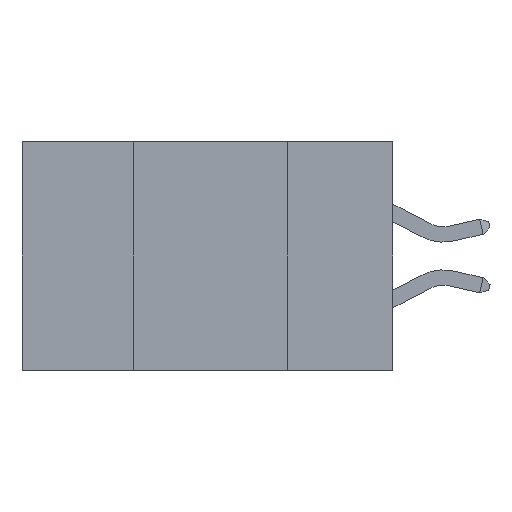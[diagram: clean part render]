
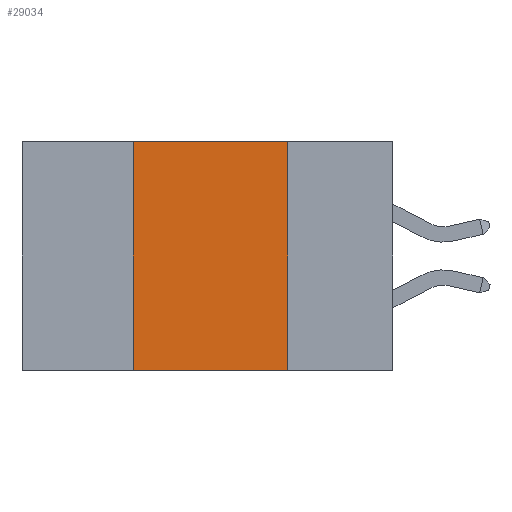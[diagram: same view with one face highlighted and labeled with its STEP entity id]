
A CAD part, left-side view. The second image highlights one B-rep face of the part: STEP entity #29034.
In plain terms, the highlighted planar face has unit normal (-1, 0, 0).
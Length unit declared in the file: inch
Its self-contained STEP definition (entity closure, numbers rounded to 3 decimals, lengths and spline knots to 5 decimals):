
#179 = CARTESIAN_POINT ( 'NONE',  ( 0., 0.17, 0. ) ) ;
#1190 = ORIENTED_EDGE ( 'NONE', *, *, #21436, .F. ) ;
#2855 = CARTESIAN_POINT ( 'NONE',  ( 0., 0.42, -0.37 ) ) ;
#4758 = CARTESIAN_POINT ( 'NONE',  ( 0., 0.6, 0. ) ) ;
#5437 = DIRECTION ( 'NONE',  ( 0., 0., -1. ) ) ;
#5873 = DIRECTION ( 'NONE',  ( 0., -1., 0. ) ) ;
#6103 = CARTESIAN_POINT ( 'NONE',  ( 0., 0.17, 0. ) ) ;
#6507 = VECTOR ( 'NONE', #5437, 39.37008 ) ;
#7411 = LINE ( 'NONE', #17559, #20046 ) ;
#9074 = ORIENTED_EDGE ( 'NONE', *, *, #22148, .F. ) ;
#9083 = ORIENTED_EDGE ( 'NONE', *, *, #24152, .F. ) ;
#9191 = AXIS2_PLACEMENT_3D ( 'NONE', #4758, #12447, #14765 ) ;
#10175 = LINE ( 'NONE', #15884, #22792 ) ;
#12447 = DIRECTION ( 'NONE',  ( 1., 0., 0. ) ) ;
#12981 = CARTESIAN_POINT ( 'NONE',  ( 0., 0.6, -0.37 ) ) ;
#13881 = VERTEX_POINT ( 'NONE', #2855 ) ;
#14174 = CARTESIAN_POINT ( 'NONE',  ( 0., 0.42, 0. ) ) ;
#14760 = LINE ( 'NONE', #179, #6507 ) ;
#14765 = DIRECTION ( 'NONE',  ( 0., 0., -1. ) ) ;
#14948 = EDGE_LOOP ( 'NONE', ( #9083, #9074, #1190, #19079 ) ) ;
#15280 = EDGE_CURVE ( 'NONE', #13881, #19726, #16064, .T. ) ;
#15884 = CARTESIAN_POINT ( 'NONE',  ( 0., 0.42, 0. ) ) ;
#16064 = LINE ( 'NONE', #12981, #19278 ) ;
#17559 = CARTESIAN_POINT ( 'NONE',  ( 0., 0.6, 0. ) ) ;
#19079 = ORIENTED_EDGE ( 'NONE', *, *, #15280, .T. ) ;
#19278 = VECTOR ( 'NONE', #25984, 39.37008 ) ;
#19669 = CARTESIAN_POINT ( 'NONE',  ( 0., 0.17, -0.37 ) ) ;
#19726 = VERTEX_POINT ( 'NONE', #19669 ) ;
#20046 = VECTOR ( 'NONE', #5873, 39.37008 ) ;
#21436 = EDGE_CURVE ( 'NONE', #13881, #31953, #10175, .T. ) ;
#22148 = EDGE_CURVE ( 'NONE', #31953, #32552, #7411, .T. ) ;
#22487 = DIRECTION ( 'NONE',  ( 0., 0., 1. ) ) ;
#22792 = VECTOR ( 'NONE', #22487, 39.37008 ) ;
#24056 = FACE_OUTER_BOUND ( 'NONE', #14948, .T. ) ;
#24152 = EDGE_CURVE ( 'NONE', #32552, #19726, #14760, .T. ) ;
#25984 = DIRECTION ( 'NONE',  ( 0., -1., 0. ) ) ;
#29034 = ADVANCED_FACE ( 'NONE', ( #24056 ), #32273, .F. ) ;
#31953 = VERTEX_POINT ( 'NONE', #14174 ) ;
#32273 = PLANE ( 'NONE',  #9191 ) ;
#32552 = VERTEX_POINT ( 'NONE', #6103 ) ;
